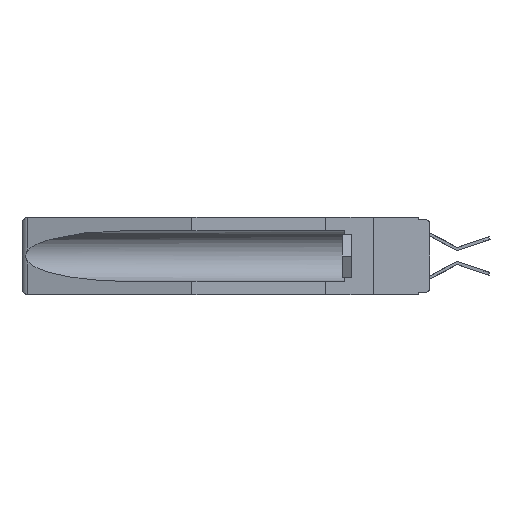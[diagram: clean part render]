
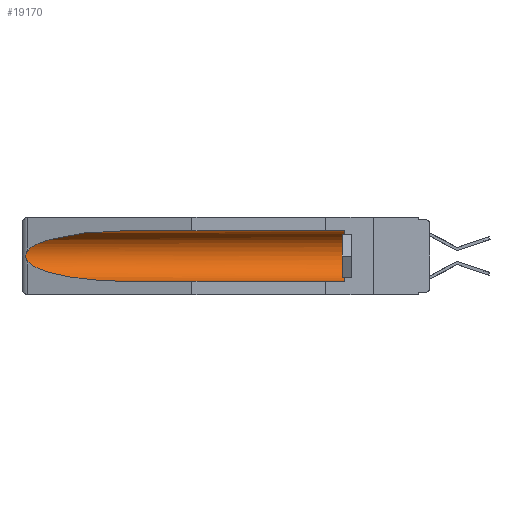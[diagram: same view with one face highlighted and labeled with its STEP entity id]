
A CAD part, left-side view. The second image highlights one B-rep face of the part: STEP entity #19170.
In plain terms, the highlighted cylindrical face has radius 2.857 mm (diameter 5.715 mm), a partial arc.
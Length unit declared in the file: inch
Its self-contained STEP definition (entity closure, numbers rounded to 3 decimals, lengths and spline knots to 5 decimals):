
#759 = ORIENTED_EDGE ( 'NONE', *, *, #7622, .T. ) ;
#1274 = DIRECTION ( 'NONE',  ( 0., 0., 1. ) ) ;
#1343 = CARTESIAN_POINT ( 'NONE',  ( 0.26537, 1.52718, -0.14972 ) ) ;
#2261 = B_SPLINE_CURVE_WITH_KNOTS ( 'NONE', 3,
 ( #18330, #2993, #5136, #24296, #16656, #8906, #7019, #22536, #10956, #8666 ),
 .UNSPECIFIED., .F., .F.,
 ( 4, 2, 2, 2, 4 ),
 ( 0., 0.00029, 0.00058, 0.00087, 0.00117 ),
 .UNSPECIFIED. ) ;
#2808 = CIRCLE ( 'NONE', #16949, 0.1125 ) ;
#2993 = CARTESIAN_POINT ( 'NONE',  ( 0.26597, 1.52961, -0.15275 ) ) ;
#3665 = LINE ( 'NONE', #11634, #4204 ) ;
#4204 = VECTOR ( 'NONE', #19381, 39.37008 ) ;
#4860 = EDGE_CURVE ( 'NONE', #6884, #16493, #7450, .T. ) ;
#5136 = CARTESIAN_POINT ( 'NONE',  ( 0.26654, 1.53092, -0.15636 ) ) ;
#5203 = EDGE_CURVE ( 'NONE', #9018, #13619, #24805, .T. ) ;
#5668 = VERTEX_POINT ( 'NONE', #9507 ) ;
#5692 = CARTESIAN_POINT ( 'NONE',  ( 0.155, 0.126, -0.284 ) ) ;
#5879 = CARTESIAN_POINT ( 'NONE',  ( 0.26537, 1.52718, -0.14972 ) ) ;
#6319 = EDGE_CURVE ( 'NONE', #13619, #6884, #2261, .T. ) ;
#6353 = ORIENTED_EDGE ( 'NONE', *, *, #18196, .T. ) ;
#6437 = DIRECTION ( 'NONE',  ( 0., 0., 1. ) ) ;
#6884 = VERTEX_POINT ( 'NONE', #25019 ) ;
#6994 = DIRECTION ( 'NONE',  ( 0., 1., 0. ) ) ;
#7019 = CARTESIAN_POINT ( 'NONE',  ( 0.2673, 1.53269, -0.17917 ) ) ;
#7073 = EDGE_LOOP ( 'NONE', ( #24201, #20649, #13607, #16846, #759, #6353 ) ) ;
#7450 =( BOUNDED_CURVE ( )  B_SPLINE_CURVE ( 3, ( #17951, #16039, #19364, #17448 ),
 .UNSPECIFIED., .F., .T. ) 
 B_SPLINE_CURVE_WITH_KNOTS ( ( 4, 4 ),
 ( 0.1948, 1.5708 ),
 .UNSPECIFIED. ) 
 CURVE ( )  GEOMETRIC_REPRESENTATION_ITEM ( )  RATIONAL_B_SPLINE_CURVE ( ( 1., 0.848, 0.848, 1. ) ) 
 REPRESENTATION_ITEM ( '' )  );
#7622 = EDGE_CURVE ( 'NONE', #15759, #5668, #2808, .T. ) ;
#8011 = CARTESIAN_POINT ( 'NONE',  ( 0.155, 1.07973, -0.059 ) ) ;
#8666 = CARTESIAN_POINT ( 'NONE',  ( 0.26537, 1.52718, -0.19328 ) ) ;
#8906 = CARTESIAN_POINT ( 'NONE',  ( 0.2675, 1.53308, -0.17534 ) ) ;
#9018 = VERTEX_POINT ( 'NONE', #8011 ) ;
#9507 = CARTESIAN_POINT ( 'NONE',  ( 0.155, 0.126, -0.059 ) ) ;
#10956 = CARTESIAN_POINT ( 'NONE',  ( 0.26597, 1.5296, -0.19026 ) ) ;
#11634 = CARTESIAN_POINT ( 'NONE',  ( 0.155, -0.30754, -0.284 ) ) ;
#12709 = LINE ( 'NONE', #16757, #19703 ) ;
#13607 = ORIENTED_EDGE ( 'NONE', *, *, #4860, .T. ) ;
#13619 = VERTEX_POINT ( 'NONE', #5879 ) ;
#15301 = FACE_OUTER_BOUND ( 'NONE', #7073, .T. ) ;
#15759 = VERTEX_POINT ( 'NONE', #5692 ) ;
#16039 = CARTESIAN_POINT ( 'NONE',  ( 0.25451, 1.48313, -0.24835 ) ) ;
#16493 = VERTEX_POINT ( 'NONE', #18441 ) ;
#16656 = CARTESIAN_POINT ( 'NONE',  ( 0.2675, 1.53308, -0.16763 ) ) ;
#16757 = CARTESIAN_POINT ( 'NONE',  ( 0.155, -0.30754, -0.059 ) ) ;
#16846 = ORIENTED_EDGE ( 'NONE', *, *, #23377, .F. ) ;
#16949 = AXIS2_PLACEMENT_3D ( 'NONE', #23717, #23961, #6437 ) ;
#16957 = DIRECTION ( 'NONE',  ( 0., 1., 0. ) ) ;
#17448 = CARTESIAN_POINT ( 'NONE',  ( 0.155, 1.07973, -0.284 ) ) ;
#17951 = CARTESIAN_POINT ( 'NONE',  ( 0.26537, 1.52718, -0.19328 ) ) ;
#18196 = EDGE_CURVE ( 'NONE', #5668, #9018, #12709, .T. ) ;
#18330 = CARTESIAN_POINT ( 'NONE',  ( 0.26537, 1.52718, -0.14972 ) ) ;
#18441 = CARTESIAN_POINT ( 'NONE',  ( 0.155, 1.07973, -0.284 ) ) ;
#19170 = ADVANCED_FACE ( 'NONE', ( #15301 ), #23059, .F. ) ;
#19203 = CARTESIAN_POINT ( 'NONE',  ( 0.21114, 1.30732, -0.059 ) ) ;
#19342 = AXIS2_PLACEMENT_3D ( 'NONE', #22937, #16957, #1274 ) ;
#19364 = CARTESIAN_POINT ( 'NONE',  ( 0.21114, 1.30732, -0.284 ) ) ;
#19381 = DIRECTION ( 'NONE',  ( 0., 1., 0. ) ) ;
#19703 = VECTOR ( 'NONE', #6994, 39.37008 ) ;
#20649 = ORIENTED_EDGE ( 'NONE', *, *, #6319, .T. ) ;
#20988 = CARTESIAN_POINT ( 'NONE',  ( 0.25451, 1.48313, -0.09465 ) ) ;
#21108 = CARTESIAN_POINT ( 'NONE',  ( 0.155, 1.07973, -0.059 ) ) ;
#22536 = CARTESIAN_POINT ( 'NONE',  ( 0.26655, 1.53094, -0.18657 ) ) ;
#22937 = CARTESIAN_POINT ( 'NONE',  ( 0.155, -0.30754, -0.1715 ) ) ;
#23059 = CYLINDRICAL_SURFACE ( 'NONE', #19342, 0.1125 ) ;
#23377 = EDGE_CURVE ( 'NONE', #15759, #16493, #3665, .T. ) ;
#23717 = CARTESIAN_POINT ( 'NONE',  ( 0.155, 0.126, -0.1715 ) ) ;
#23961 = DIRECTION ( 'NONE',  ( 0., -1., 0. ) ) ;
#24201 = ORIENTED_EDGE ( 'NONE', *, *, #5203, .T. ) ;
#24296 = CARTESIAN_POINT ( 'NONE',  ( 0.2673, 1.5327, -0.16383 ) ) ;
#24805 =( BOUNDED_CURVE ( )  B_SPLINE_CURVE ( 3, ( #21108, #19203, #20988, #1343 ),
 .UNSPECIFIED., .F., .T. ) 
 B_SPLINE_CURVE_WITH_KNOTS ( ( 4, 4 ),
 ( 4.71239, 6.08839 ),
 .UNSPECIFIED. ) 
 CURVE ( )  GEOMETRIC_REPRESENTATION_ITEM ( )  RATIONAL_B_SPLINE_CURVE ( ( 1., 0.848, 0.848, 1. ) ) 
 REPRESENTATION_ITEM ( '' )  );
#25019 = CARTESIAN_POINT ( 'NONE',  ( 0.26537, 1.52718, -0.19328 ) ) ;
